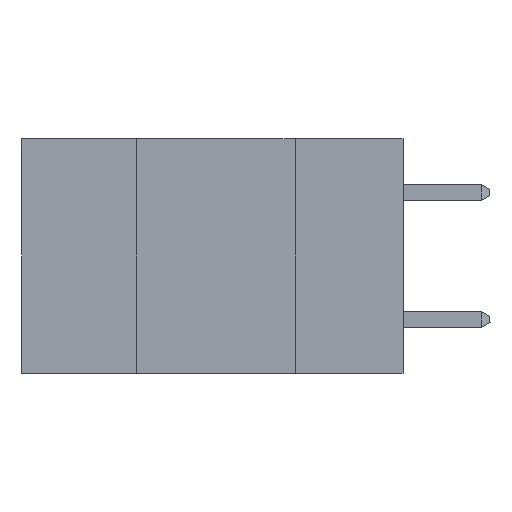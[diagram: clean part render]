
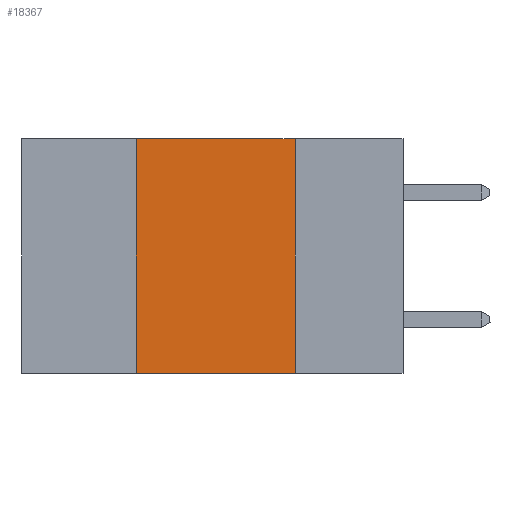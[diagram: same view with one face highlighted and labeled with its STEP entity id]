
A CAD part, left-side view. The second image highlights one B-rep face of the part: STEP entity #18367.
In plain terms, the highlighted planar face has unit normal (-1, 0, 0).
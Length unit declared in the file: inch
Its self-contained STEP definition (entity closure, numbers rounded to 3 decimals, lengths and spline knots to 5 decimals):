
#177 = ORIENTED_EDGE ( 'NONE', *, *, #3291, .F. ) ;
#1044 = VERTEX_POINT ( 'NONE', #8473 ) ;
#2752 = EDGE_CURVE ( 'NONE', #12207, #25026, #11723, .T. ) ;
#2935 = LINE ( 'NONE', #26757, #6561 ) ;
#3222 = AXIS2_PLACEMENT_3D ( 'NONE', #9057, #17433, #17254 ) ;
#3291 = EDGE_CURVE ( 'NONE', #12207, #1044, #16970, .T. ) ;
#4025 = CARTESIAN_POINT ( 'NONE',  ( 0., 0.17, 0. ) ) ;
#4633 = VECTOR ( 'NONE', #18639, 39.37008 ) ;
#5882 = CARTESIAN_POINT ( 'NONE',  ( 0., 0.42, 0. ) ) ;
#6561 = VECTOR ( 'NONE', #20556, 39.37008 ) ;
#6929 = CARTESIAN_POINT ( 'NONE',  ( 0., 0.17, 0. ) ) ;
#7572 = VERTEX_POINT ( 'NONE', #6929 ) ;
#8473 = CARTESIAN_POINT ( 'NONE',  ( 0., 0.42, 0. ) ) ;
#9057 = CARTESIAN_POINT ( 'NONE',  ( 0., 0.6, 0. ) ) ;
#10115 = DIRECTION ( 'NONE',  ( 0., 0., 1. ) ) ;
#10363 = VECTOR ( 'NONE', #10115, 39.37008 ) ;
#11723 = LINE ( 'NONE', #17621, #15336 ) ;
#12207 = VERTEX_POINT ( 'NONE', #25971 ) ;
#13203 = DIRECTION ( 'NONE',  ( 0., -1., 0. ) ) ;
#14178 = ORIENTED_EDGE ( 'NONE', *, *, #16075, .F. ) ;
#15190 = ORIENTED_EDGE ( 'NONE', *, *, #21455, .F. ) ;
#15336 = VECTOR ( 'NONE', #13203, 39.37008 ) ;
#16075 = EDGE_CURVE ( 'NONE', #7572, #25026, #20720, .T. ) ;
#16970 = LINE ( 'NONE', #5882, #10363 ) ;
#17254 = DIRECTION ( 'NONE',  ( 0., 0., -1. ) ) ;
#17433 = DIRECTION ( 'NONE',  ( 1., 0., 0. ) ) ;
#17621 = CARTESIAN_POINT ( 'NONE',  ( 0., 0.6, -0.37 ) ) ;
#18367 = ADVANCED_FACE ( 'NONE', ( #23160 ), #21359, .F. ) ;
#18639 = DIRECTION ( 'NONE',  ( 0., 0., -1. ) ) ;
#20556 = DIRECTION ( 'NONE',  ( 0., -1., 0. ) ) ;
#20720 = LINE ( 'NONE', #4025, #4633 ) ;
#20988 = CARTESIAN_POINT ( 'NONE',  ( 0., 0.17, -0.37 ) ) ;
#21359 = PLANE ( 'NONE',  #3222 ) ;
#21455 = EDGE_CURVE ( 'NONE', #1044, #7572, #2935, .T. ) ;
#21591 = EDGE_LOOP ( 'NONE', ( #14178, #15190, #177, #27081 ) ) ;
#23160 = FACE_OUTER_BOUND ( 'NONE', #21591, .T. ) ;
#25026 = VERTEX_POINT ( 'NONE', #20988 ) ;
#25971 = CARTESIAN_POINT ( 'NONE',  ( 0., 0.42, -0.37 ) ) ;
#26757 = CARTESIAN_POINT ( 'NONE',  ( 0., 0.6, 0. ) ) ;
#27081 = ORIENTED_EDGE ( 'NONE', *, *, #2752, .T. ) ;
